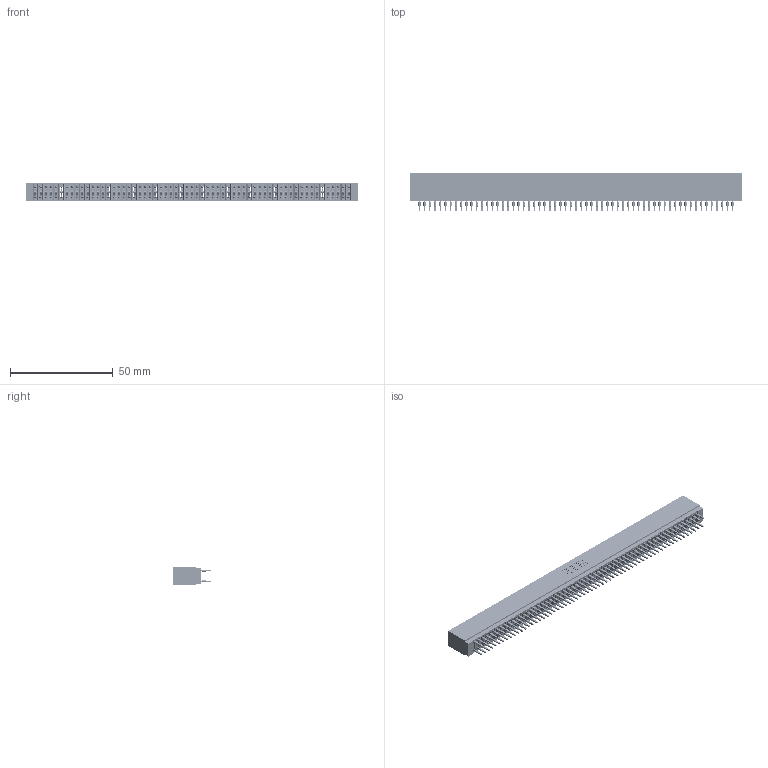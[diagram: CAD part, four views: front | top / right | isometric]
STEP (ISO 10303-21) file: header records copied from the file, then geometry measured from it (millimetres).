
FILE_DESCRIPTION (( 'STEP AP203' ), '1' );
FILE_NAME ('725-122-560-201.STEP', '2026-02-24T21:12:59', ( '' ), ( '' ), 'SwSTEP 2.0', 'SolidWorks 2023', '' );
FILE_SCHEMA (( 'CONFIG_CONTROL_DESIGN' ));
Products named in the file (3): 725 Part_Insulator Option - 01; 745-292-001_560; 725-122-560-201
Assembly tree (123 placements, depth 2):
  725-122-560-201
    725 Part_Insulator Option - 01
    745-292-001_560  x122
Bounding box: 161.54 x 18.8 x 8.89 mm (x, y, z)
Volume: 13165.6 mm3; surface area: 30137.3 mm2
Topology: 123 solids, 123 shells, 12112 faces, 33133 edges, 21030 vertices
Faces by surface type: plane 6277, cylinder 2663, bspline 2440, torus 732
Entity records: 100388 total; most frequent: CARTESIAN_POINT 17909, ORIENTED_EDGE 17382, DIRECTION 15175, EDGE_CURVE 8691, LINE 8135, VECTOR 8135, VERTEX_POINT 5542, AXIS2_PLACEMENT_3D 3520
